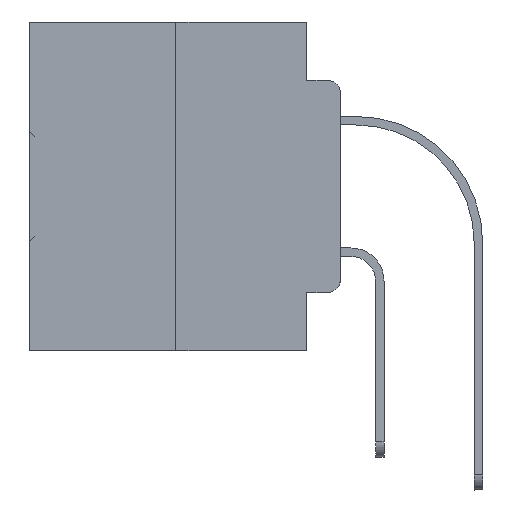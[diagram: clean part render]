
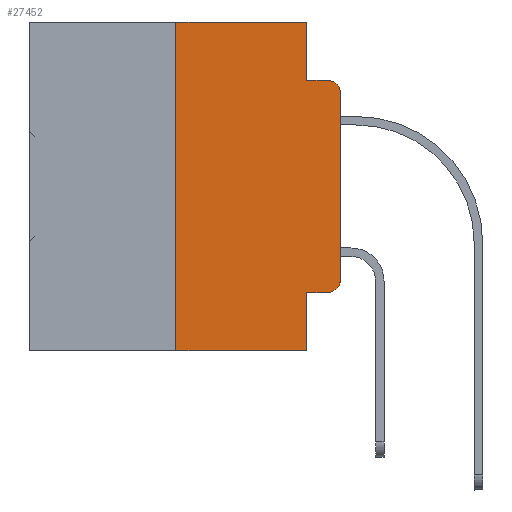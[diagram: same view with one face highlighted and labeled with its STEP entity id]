
A CAD part, left-side view. The second image highlights one B-rep face of the part: STEP entity #27452.
In plain terms, the highlighted planar face has unit normal (-1, 0, 0).
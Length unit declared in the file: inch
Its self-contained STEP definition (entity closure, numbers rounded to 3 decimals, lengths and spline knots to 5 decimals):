
#229 = VECTOR ( 'NONE', #19196, 39.37008 ) ;
#506 = EDGE_CURVE ( 'NONE', #22332, #17918, #18046, .T. ) ;
#545 = CARTESIAN_POINT ( 'NONE',  ( 0., 0.02, -0.0885 ) ) ;
#1153 = EDGE_CURVE ( 'NONE', #14091, #1735, #34878, .T. ) ;
#1347 = CARTESIAN_POINT ( 'NONE',  ( 0., 0.473, 0. ) ) ;
#1735 = VERTEX_POINT ( 'NONE', #8467 ) ;
#2176 = ORIENTED_EDGE ( 'NONE', *, *, #34035, .F. ) ;
#2222 = VECTOR ( 'NONE', #3051, 39.37008 ) ;
#2580 = DIRECTION ( 'NONE',  ( 0., -1., 0. ) ) ;
#2640 = LINE ( 'NONE', #19768, #17898 ) ;
#2769 = DIRECTION ( 'NONE',  ( 0., 0., -1. ) ) ;
#3051 = DIRECTION ( 'NONE',  ( 0., -1., 0. ) ) ;
#3422 = ORIENTED_EDGE ( 'NONE', *, *, #32720, .T. ) ;
#4234 = EDGE_CURVE ( 'NONE', #1735, #12758, #19674, .T. ) ;
#4431 = PLANE ( 'NONE',  #18523 ) ;
#4754 = CARTESIAN_POINT ( 'NONE',  ( 0., 0.051, -0.5 ) ) ;
#5862 = LINE ( 'NONE', #31843, #35955 ) ;
#8182 = LINE ( 'NONE', #22798, #24403 ) ;
#8467 = CARTESIAN_POINT ( 'NONE',  ( 0., 0.051, -0.0885 ) ) ;
#8998 = ORIENTED_EDGE ( 'NONE', *, *, #34777, .F. ) ;
#10143 = CIRCLE ( 'NONE', #14410, 0.02 ) ;
#10365 = CARTESIAN_POINT ( 'NONE',  ( 0., 0.02, -0.3915 ) ) ;
#10522 = ORIENTED_EDGE ( 'NONE', *, *, #27082, .T. ) ;
#10560 = LINE ( 'NONE', #19380, #16359 ) ;
#10962 = ORIENTED_EDGE ( 'NONE', *, *, #33563, .T. ) ;
#11789 = CARTESIAN_POINT ( 'NONE',  ( 0., 0.051, 0. ) ) ;
#11956 = DIRECTION ( 'NONE',  ( -1., 0., 0. ) ) ;
#12564 = ORIENTED_EDGE ( 'NONE', *, *, #12935, .F. ) ;
#12758 = VERTEX_POINT ( 'NONE', #545 ) ;
#12935 = EDGE_CURVE ( 'NONE', #22332, #34494, #25186, .T. ) ;
#13101 = DIRECTION ( 'NONE',  ( 1., 0., 0. ) ) ;
#14091 = VERTEX_POINT ( 'NONE', #11789 ) ;
#14095 = CARTESIAN_POINT ( 'NONE',  ( 0., 0.051, 0. ) ) ;
#14361 = VERTEX_POINT ( 'NONE', #19254 ) ;
#14410 = AXIS2_PLACEMENT_3D ( 'NONE', #10365, #19936, #14558 ) ;
#14558 = DIRECTION ( 'NONE',  ( 0., 0., -1. ) ) ;
#15686 = CARTESIAN_POINT ( 'NONE',  ( 0., 0.25, -0.5 ) ) ;
#16336 = EDGE_LOOP ( 'NONE', ( #10522, #3422, #24968, #27028, #8998, #12564, #17915, #2176, #28733, #10962 ) ) ;
#16359 = VECTOR ( 'NONE', #24792, 39.37008 ) ;
#16690 = CARTESIAN_POINT ( 'NONE',  ( 0., 0.25, 0. ) ) ;
#16973 = CARTESIAN_POINT ( 'NONE',  ( 0., 0., -0.1085 ) ) ;
#17898 = VECTOR ( 'NONE', #31911, 39.37008 ) ;
#17911 = DIRECTION ( 'NONE',  ( 0., 0., -1. ) ) ;
#17915 = ORIENTED_EDGE ( 'NONE', *, *, #506, .T. ) ;
#17918 = VERTEX_POINT ( 'NONE', #4754 ) ;
#18046 = LINE ( 'NONE', #26341, #2222 ) ;
#18523 = AXIS2_PLACEMENT_3D ( 'NONE', #1347, #13101, #36589 ) ;
#19196 = DIRECTION ( 'NONE',  ( 0., 0., 1. ) ) ;
#19254 = CARTESIAN_POINT ( 'NONE',  ( 0., 0., -0.3915 ) ) ;
#19380 = CARTESIAN_POINT ( 'NONE',  ( 0., 0.473, 0. ) ) ;
#19674 = LINE ( 'NONE', #23142, #25199 ) ;
#19768 = CARTESIAN_POINT ( 'NONE',  ( 0., 0., 0. ) ) ;
#19936 = DIRECTION ( 'NONE',  ( -1., 0., 0. ) ) ;
#20389 = VERTEX_POINT ( 'NONE', #31933 ) ;
#20438 = DIRECTION ( 'NONE',  ( 0., -1., 0. ) ) ;
#21733 = AXIS2_PLACEMENT_3D ( 'NONE', #26568, #11956, #17911 ) ;
#22332 = VERTEX_POINT ( 'NONE', #15686 ) ;
#22798 = CARTESIAN_POINT ( 'NONE',  ( 0., 0.051, -0.4115 ) ) ;
#23081 = VERTEX_POINT ( 'NONE', #16973 ) ;
#23142 = CARTESIAN_POINT ( 'NONE',  ( 0., 0.051, -0.0885 ) ) ;
#24382 = EDGE_CURVE ( 'NONE', #20389, #33963, #8182, .T. ) ;
#24403 = VECTOR ( 'NONE', #2580, 39.37008 ) ;
#24456 = FACE_OUTER_BOUND ( 'NONE', #16336, .T. ) ;
#24792 = DIRECTION ( 'NONE',  ( 0., -1., 0. ) ) ;
#24968 = ORIENTED_EDGE ( 'NONE', *, *, #4234, .F. ) ;
#25186 = LINE ( 'NONE', #16690, #229 ) ;
#25199 = VECTOR ( 'NONE', #20438, 39.37008 ) ;
#26341 = CARTESIAN_POINT ( 'NONE',  ( 0., 0.473, -0.5 ) ) ;
#26568 = CARTESIAN_POINT ( 'NONE',  ( 0., 0.02, -0.1085 ) ) ;
#27028 = ORIENTED_EDGE ( 'NONE', *, *, #1153, .F. ) ;
#27082 = EDGE_CURVE ( 'NONE', #14361, #23081, #2640, .T. ) ;
#27452 = ADVANCED_FACE ( 'NONE', ( #24456 ), #4431, .F. ) ;
#28200 = CARTESIAN_POINT ( 'NONE',  ( 0., 0.02, -0.4115 ) ) ;
#28340 = DIRECTION ( 'NONE',  ( 0., 0., -1. ) ) ;
#28372 = VECTOR ( 'NONE', #28340, 39.37008 ) ;
#28733 = ORIENTED_EDGE ( 'NONE', *, *, #24382, .T. ) ;
#31425 = CARTESIAN_POINT ( 'NONE',  ( 0., 0.25, 0. ) ) ;
#31843 = CARTESIAN_POINT ( 'NONE',  ( 0., 0.051, 0. ) ) ;
#31911 = DIRECTION ( 'NONE',  ( 0., 0., 1. ) ) ;
#31933 = CARTESIAN_POINT ( 'NONE',  ( 0., 0.051, -0.4115 ) ) ;
#32196 = CIRCLE ( 'NONE', #21733, 0.02 ) ;
#32720 = EDGE_CURVE ( 'NONE', #23081, #12758, #32196, .T. ) ;
#33563 = EDGE_CURVE ( 'NONE', #33963, #14361, #10143, .T. ) ;
#33963 = VERTEX_POINT ( 'NONE', #28200 ) ;
#34035 = EDGE_CURVE ( 'NONE', #20389, #17918, #5862, .T. ) ;
#34494 = VERTEX_POINT ( 'NONE', #31425 ) ;
#34777 = EDGE_CURVE ( 'NONE', #34494, #14091, #10560, .T. ) ;
#34878 = LINE ( 'NONE', #14095, #28372 ) ;
#35955 = VECTOR ( 'NONE', #2769, 39.37008 ) ;
#36589 = DIRECTION ( 'NONE',  ( 0., 0., -1. ) ) ;
